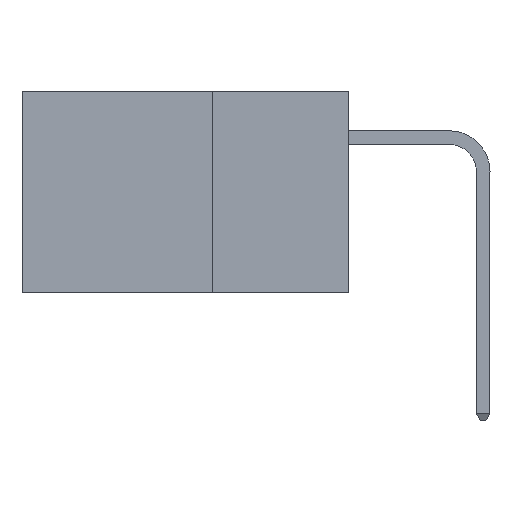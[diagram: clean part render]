
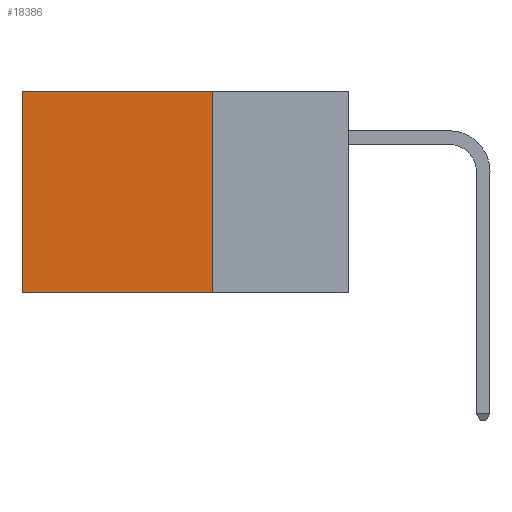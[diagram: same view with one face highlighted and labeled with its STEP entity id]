
A CAD part, left-side view. The second image highlights one B-rep face of the part: STEP entity #18386.
In plain terms, the highlighted planar face has unit normal (-1, 0, 0).
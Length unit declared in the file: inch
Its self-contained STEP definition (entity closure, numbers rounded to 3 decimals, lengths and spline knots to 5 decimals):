
#754 = CARTESIAN_POINT ( 'NONE',  ( 0.2875, 0.6, 0. ) ) ;
#1178 = EDGE_LOOP ( 'NONE', ( #1860, #5440, #9251, #4921 ) ) ;
#1259 = VERTEX_POINT ( 'NONE', #6836 ) ;
#1516 = CARTESIAN_POINT ( 'NONE',  ( 0.2875, 0.6, -0.37 ) ) ;
#1617 = CARTESIAN_POINT ( 'NONE',  ( 0.2875, 0.25, 0. ) ) ;
#1860 = ORIENTED_EDGE ( 'NONE', *, *, #3148, .T. ) ;
#2063 = DIRECTION ( 'NONE',  ( 1., 0., 0. ) ) ;
#3148 = EDGE_CURVE ( 'NONE', #11559, #19122, #14368, .T. ) ;
#3492 = EDGE_CURVE ( 'NONE', #11280, #1259, #12229, .T. ) ;
#4629 = AXIS2_PLACEMENT_3D ( 'NONE', #17367, #2063, #12850 ) ;
#4921 = ORIENTED_EDGE ( 'NONE', *, *, #8879, .T. ) ;
#5440 = ORIENTED_EDGE ( 'NONE', *, *, #8136, .F. ) ;
#6703 = LINE ( 'NONE', #18391, #14277 ) ;
#6731 = DIRECTION ( 'NONE',  ( 0., 0., -1. ) ) ;
#6836 = CARTESIAN_POINT ( 'NONE',  ( 0.2875, 0.25, -0.37 ) ) ;
#7913 = VECTOR ( 'NONE', #12778, 39.37008 ) ;
#8136 = EDGE_CURVE ( 'NONE', #1259, #19122, #6703, .T. ) ;
#8243 = VECTOR ( 'NONE', #18623, 39.37008 ) ;
#8879 = EDGE_CURVE ( 'NONE', #11280, #11559, #19522, .T. ) ;
#9251 = ORIENTED_EDGE ( 'NONE', *, *, #3492, .F. ) ;
#10113 = CARTESIAN_POINT ( 'NONE',  ( 0.2875, 0.6, 0. ) ) ;
#11280 = VERTEX_POINT ( 'NONE', #1617 ) ;
#11343 = PLANE ( 'NONE',  #4629 ) ;
#11559 = VERTEX_POINT ( 'NONE', #10113 ) ;
#12229 = LINE ( 'NONE', #16366, #8243 ) ;
#12778 = DIRECTION ( 'NONE',  ( 0., 1., 0. ) ) ;
#12850 = DIRECTION ( 'NONE',  ( 0., 0., -1. ) ) ;
#13904 = VECTOR ( 'NONE', #6731, 39.37008 ) ;
#14277 = VECTOR ( 'NONE', #16863, 39.37008 ) ;
#14368 = LINE ( 'NONE', #754, #13904 ) ;
#16366 = CARTESIAN_POINT ( 'NONE',  ( 0.2875, 0.25, 0. ) ) ;
#16863 = DIRECTION ( 'NONE',  ( 0., 1., 0. ) ) ;
#17073 = FACE_OUTER_BOUND ( 'NONE', #1178, .T. ) ;
#17367 = CARTESIAN_POINT ( 'NONE',  ( 0.2875, 0.25, 0. ) ) ;
#18386 = ADVANCED_FACE ( 'NONE', ( #17073 ), #11343, .F. ) ;
#18391 = CARTESIAN_POINT ( 'NONE',  ( 0.2875, 0.25, -0.37 ) ) ;
#18623 = DIRECTION ( 'NONE',  ( 0., 0., -1. ) ) ;
#18829 = CARTESIAN_POINT ( 'NONE',  ( 0.2875, 0.25, 0. ) ) ;
#19122 = VERTEX_POINT ( 'NONE', #1516 ) ;
#19522 = LINE ( 'NONE', #18829, #7913 ) ;
